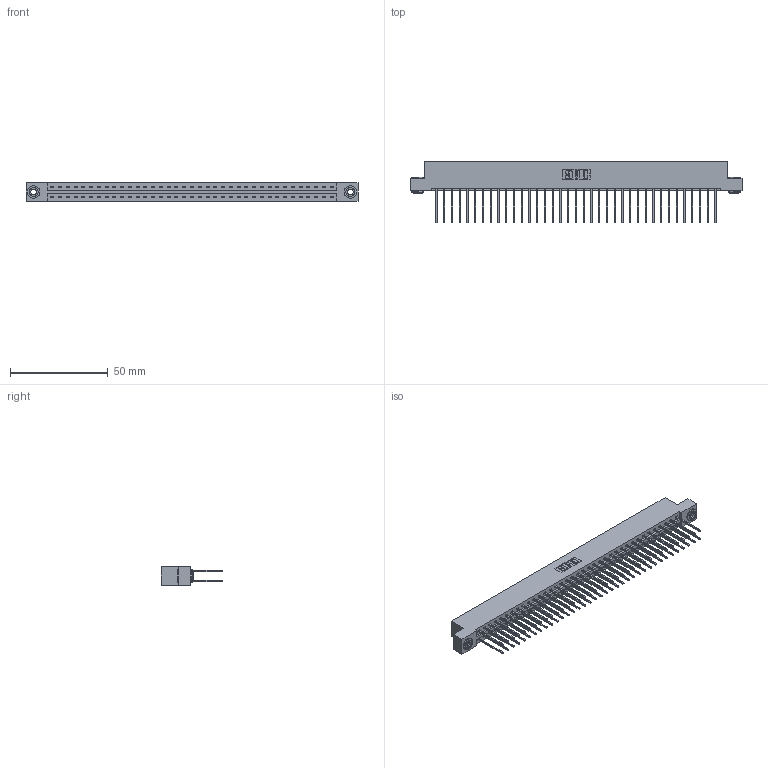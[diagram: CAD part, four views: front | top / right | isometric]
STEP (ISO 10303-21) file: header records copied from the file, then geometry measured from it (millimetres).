
FILE_DESCRIPTION (( 'STEP AP203' ), '1' );
FILE_NAME ('387-074-542-203.STEP', '2018-09-22T19:59:12', ( '' ), ( '' ), 'SwSTEP 2.0', 'SolidWorks 2016', '' );
FILE_SCHEMA (( 'CONFIG_CONTROL_DESIGN' ));
Length unit declared in the file: inch
Products named in the file (4): 345-292-001_345-293-142; 345-250-002_345-250-002-102; 387-074-542-203; 337 Part_Flush Mounting Lugs - 0.156 Dia-TH
Assembly tree (77 placements, depth 2):
  387-074-542-203
    337 Part_Flush Mounting Lugs - 0.156 Dia-TH
    345-292-001_345-293-142  x74
    345-250-002_345-250-002-102  x2
Bounding box: 169.62 x 31.63 x 9.4 mm (x, y, z)
Volume: 18173.8 mm3; surface area: 22441.1 mm2
Topology: 77 solids, 77 shells, 4148 faces, 12301 edges, 8098 vertices
Faces by surface type: plane 2892, cylinder 1248, cone 8
Entity records: 30002 total; most frequent: CARTESIAN_POINT 5033, ORIENTED_EDGE 4962, DIRECTION 4323, EDGE_CURVE 2481, VECTOR 2329, LINE 2329, VERTEX_POINT 1650, AXIS2_PLACEMENT_3D 997
